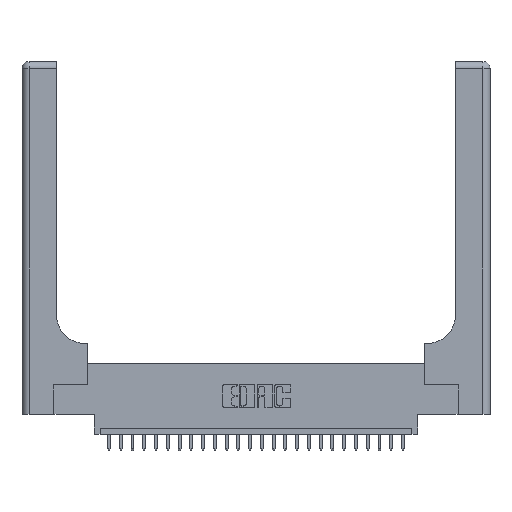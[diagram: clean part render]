
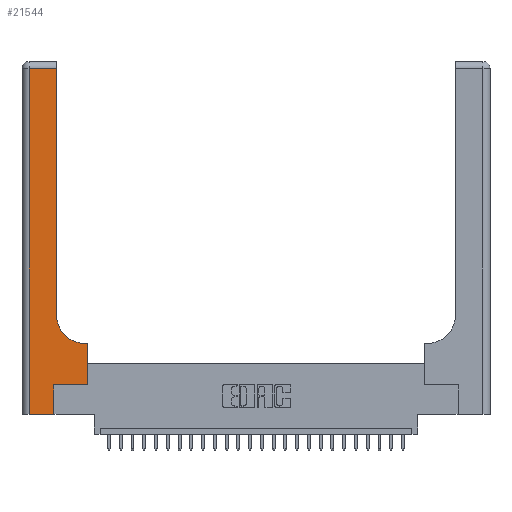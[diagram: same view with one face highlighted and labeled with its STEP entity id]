
A CAD part, top view. The second image highlights one B-rep face of the part: STEP entity #21544.
In plain terms, the highlighted planar face has unit normal (0, 0, 1).
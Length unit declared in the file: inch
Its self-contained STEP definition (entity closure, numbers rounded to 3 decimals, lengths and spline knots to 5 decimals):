
#73 = DIRECTION ( 'NONE',  ( -1., 0., 0. ) ) ;
#161 = CARTESIAN_POINT ( 'NONE',  ( 0., 2.94, 0.37 ) ) ;
#739 = CARTESIAN_POINT ( 'NONE',  ( 0.269, 0., 0.37 ) ) ;
#822 = ORIENTED_EDGE ( 'NONE', *, *, #10188, .T. ) ;
#1259 = VECTOR ( 'NONE', #73, 39.37008 ) ;
#1376 = ORIENTED_EDGE ( 'NONE', *, *, #5176, .T. ) ;
#1595 = FACE_OUTER_BOUND ( 'NONE', #20583, .T. ) ;
#2153 = CARTESIAN_POINT ( 'NONE',  ( 0.5585, 0.25, 0.37 ) ) ;
#2411 = ORIENTED_EDGE ( 'NONE', *, *, #11625, .T. ) ;
#2554 = DIRECTION ( 'NONE',  ( 0., 1., 0. ) ) ;
#2650 = DIRECTION ( 'NONE',  ( 0., 1., 0. ) ) ;
#2801 = CARTESIAN_POINT ( 'NONE',  ( 0.06, 0., 0.37 ) ) ;
#3209 = VECTOR ( 'NONE', #2554, 39.37008 ) ;
#3844 = AXIS2_PLACEMENT_3D ( 'NONE', #5493, #12059, #7613 ) ;
#4094 = VERTEX_POINT ( 'NONE', #16953 ) ;
#4534 = CARTESIAN_POINT ( 'NONE',  ( 0., 0., 0.37 ) ) ;
#4974 = DIRECTION ( 'NONE',  ( 0., 0., -1. ) ) ;
#5176 = EDGE_CURVE ( 'NONE', #20678, #10348, #18598, .T. ) ;
#5342 = CARTESIAN_POINT ( 'NONE',  ( 0.2915, 3., 0.37 ) ) ;
#5470 = EDGE_CURVE ( 'NONE', #11404, #23060, #16280, .T. ) ;
#5493 = CARTESIAN_POINT ( 'NONE',  ( 0.5415, 0.85, 0.37 ) ) ;
#5614 = VECTOR ( 'NONE', #22515, 39.37008 ) ;
#6519 = PLANE ( 'NONE',  #22036 ) ;
#7083 = CARTESIAN_POINT ( 'NONE',  ( 0.269, 0., 0.37 ) ) ;
#7118 = CARTESIAN_POINT ( 'NONE',  ( 0.269, 0.25, 0.37 ) ) ;
#7513 = LINE ( 'NONE', #5342, #15988 ) ;
#7613 = DIRECTION ( 'NONE',  ( 1., 0., 0. ) ) ;
#8381 = LINE ( 'NONE', #7118, #20106 ) ;
#9467 = CARTESIAN_POINT ( 'NONE',  ( 0.5415, 0.6, 0.37 ) ) ;
#9944 = CARTESIAN_POINT ( 'NONE',  ( 0.06, 3., 0.37 ) ) ;
#10188 = EDGE_CURVE ( 'NONE', #12269, #15414, #11090, .T. ) ;
#10230 = EDGE_CURVE ( 'NONE', #15414, #22672, #7513, .T. ) ;
#10348 = VERTEX_POINT ( 'NONE', #2801 ) ;
#10573 = CARTESIAN_POINT ( 'NONE',  ( 0.06, 2.94, 0.37 ) ) ;
#10968 = CARTESIAN_POINT ( 'NONE',  ( 0.5585, 0.25, 0.37 ) ) ;
#11037 = LINE ( 'NONE', #7083, #17560 ) ;
#11064 = EDGE_CURVE ( 'NONE', #19544, #4094, #11037, .T. ) ;
#11090 = CIRCLE ( 'NONE', #3844, 0.25 ) ;
#11198 = ORIENTED_EDGE ( 'NONE', *, *, #12484, .T. ) ;
#11404 = VERTEX_POINT ( 'NONE', #2153 ) ;
#11625 = EDGE_CURVE ( 'NONE', #4094, #11404, #8381, .T. ) ;
#11822 = LINE ( 'NONE', #13469, #5614 ) ;
#12059 = DIRECTION ( 'NONE',  ( 0., 0., -1. ) ) ;
#12269 = VERTEX_POINT ( 'NONE', #9467 ) ;
#12321 = DIRECTION ( 'NONE',  ( 0., -1., 0. ) ) ;
#12454 = ORIENTED_EDGE ( 'NONE', *, *, #21840, .T. ) ;
#12484 = EDGE_CURVE ( 'NONE', #10348, #19544, #25621, .T. ) ;
#13469 = CARTESIAN_POINT ( 'NONE',  ( 0.2915, 0.6, 0.37 ) ) ;
#13497 = ORIENTED_EDGE ( 'NONE', *, *, #11064, .T. ) ;
#15343 = CARTESIAN_POINT ( 'NONE',  ( 0.2915, 2.94, 0.37 ) ) ;
#15414 = VERTEX_POINT ( 'NONE', #17257 ) ;
#15988 = VECTOR ( 'NONE', #2650, 39.37008 ) ;
#15999 = LINE ( 'NONE', #161, #1259 ) ;
#16280 = LINE ( 'NONE', #10968, #3209 ) ;
#16953 = CARTESIAN_POINT ( 'NONE',  ( 0.269, 0.25, 0.37 ) ) ;
#17257 = CARTESIAN_POINT ( 'NONE',  ( 0.2915, 0.85, 0.37 ) ) ;
#17560 = VECTOR ( 'NONE', #23628, 39.37008 ) ;
#17562 = DIRECTION ( 'NONE',  ( -1., 0., 0. ) ) ;
#18122 = VECTOR ( 'NONE', #25120, 39.37008 ) ;
#18484 = EDGE_CURVE ( 'NONE', #23060, #12269, #11822, .T. ) ;
#18598 = LINE ( 'NONE', #9944, #18938 ) ;
#18938 = VECTOR ( 'NONE', #12321, 39.37008 ) ;
#19192 = CARTESIAN_POINT ( 'NONE',  ( 0., 3., 0.37 ) ) ;
#19544 = VERTEX_POINT ( 'NONE', #739 ) ;
#20040 = ORIENTED_EDGE ( 'NONE', *, *, #10230, .T. ) ;
#20106 = VECTOR ( 'NONE', #25972, 39.37008 ) ;
#20583 = EDGE_LOOP ( 'NONE', ( #20040, #12454, #1376, #11198, #13497, #2411, #21841, #26870, #822 ) ) ;
#20678 = VERTEX_POINT ( 'NONE', #10573 ) ;
#21544 = ADVANCED_FACE ( 'NONE', ( #1595 ), #6519, .F. ) ;
#21840 = EDGE_CURVE ( 'NONE', #22672, #20678, #15999, .T. ) ;
#21841 = ORIENTED_EDGE ( 'NONE', *, *, #5470, .T. ) ;
#22036 = AXIS2_PLACEMENT_3D ( 'NONE', #19192, #4974, #17562 ) ;
#22515 = DIRECTION ( 'NONE',  ( -1., 0., 0. ) ) ;
#22672 = VERTEX_POINT ( 'NONE', #15343 ) ;
#23060 = VERTEX_POINT ( 'NONE', #24523 ) ;
#23628 = DIRECTION ( 'NONE',  ( 0., 1., 0. ) ) ;
#24523 = CARTESIAN_POINT ( 'NONE',  ( 0.5585, 0.6, 0.37 ) ) ;
#25120 = DIRECTION ( 'NONE',  ( 1., 0., 0. ) ) ;
#25621 = LINE ( 'NONE', #4534, #18122 ) ;
#25972 = DIRECTION ( 'NONE',  ( 1., 0., 0. ) ) ;
#26870 = ORIENTED_EDGE ( 'NONE', *, *, #18484, .T. ) ;
